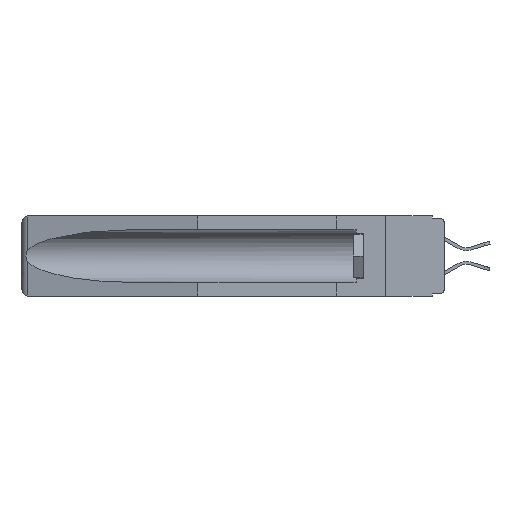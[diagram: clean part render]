
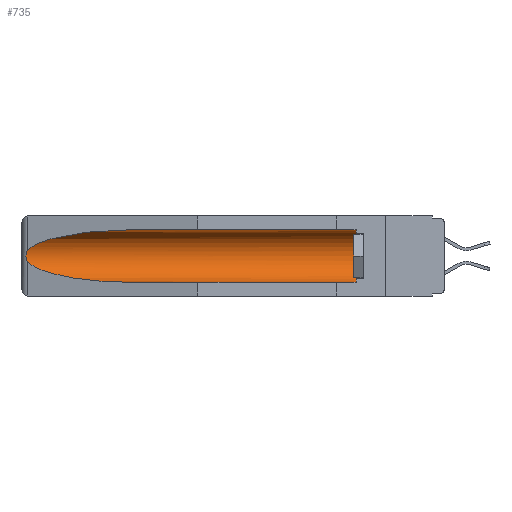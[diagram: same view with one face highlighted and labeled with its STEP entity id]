
A CAD part, left-side view. The second image highlights one B-rep face of the part: STEP entity #735.
In plain terms, the highlighted cylindrical face has radius 2.857 mm (diameter 5.715 mm), a partial arc.
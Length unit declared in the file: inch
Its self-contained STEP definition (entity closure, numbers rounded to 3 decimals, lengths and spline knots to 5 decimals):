
#146 = ORIENTED_EDGE ( 'NONE', *, *, #21408, .T. ) ;
#320 = EDGE_CURVE ( 'NONE', #24030, #10527, #571, .T. ) ;
#353 = CARTESIAN_POINT ( 'NONE',  ( 0.155, 1.07973, -0.284 ) ) ;
#571 = LINE ( 'NONE', #12429, #3613 ) ;
#735 = ADVANCED_FACE ( 'NONE', ( #6229 ), #23232, .F. ) ;
#1528 = CARTESIAN_POINT ( 'NONE',  ( 0.155, 1.07973, -0.284 ) ) ;
#1650 = CARTESIAN_POINT ( 'NONE',  ( 0.26537, 1.52718, -0.19328 ) ) ;
#1743 = CARTESIAN_POINT ( 'NONE',  ( 0.26597, 1.5296, -0.19026 ) ) ;
#1831 = B_SPLINE_CURVE_WITH_KNOTS ( 'NONE', 3,
 ( #9796, #8212, #12398, #12588, #23132, #27302, #14442, #27588, #1743, #1650 ),
 .UNSPECIFIED., .F., .F.,
 ( 4, 2, 2, 2, 4 ),
 ( 0., 0.00029, 0.00058, 0.00087, 0.00117 ),
 .UNSPECIFIED. ) ;
#3613 = VECTOR ( 'NONE', #27330, 39.37008 ) ;
#4956 = AXIS2_PLACEMENT_3D ( 'NONE', #20305, #7686, #22419 ) ;
#5510 = ORIENTED_EDGE ( 'NONE', *, *, #18144, .T. ) ;
#6229 = FACE_OUTER_BOUND ( 'NONE', #10276, .T. ) ;
#6722 = CARTESIAN_POINT ( 'NONE',  ( 0.26537, 1.52718, -0.14972 ) ) ;
#6741 = ORIENTED_EDGE ( 'NONE', *, *, #320, .T. ) ;
#7222 = VERTEX_POINT ( 'NONE', #6722 ) ;
#7345 =( BOUNDED_CURVE ( )  B_SPLINE_CURVE ( 3, ( #22828, #18280, #24866, #1528 ),
 .UNSPECIFIED., .F., .F. ) 
 B_SPLINE_CURVE_WITH_KNOTS ( ( 4, 4 ),
 ( 0.1948, 1.5708 ),
 .UNSPECIFIED. ) 
 CURVE ( )  GEOMETRIC_REPRESENTATION_ITEM ( )  RATIONAL_B_SPLINE_CURVE ( ( 1., 0.848, 0.848, 1. ) ) 
 REPRESENTATION_ITEM ( '' )  );
#7449 = CARTESIAN_POINT ( 'NONE',  ( 0.155, 0.126, -0.284 ) ) ;
#7686 = DIRECTION ( 'NONE',  ( 0., 1., 0. ) ) ;
#8075 = CARTESIAN_POINT ( 'NONE',  ( 0.21114, 1.30732, -0.059 ) ) ;
#8212 = CARTESIAN_POINT ( 'NONE',  ( 0.26597, 1.52961, -0.15275 ) ) ;
#8439 = LINE ( 'NONE', #22333, #11443 ) ;
#9251 = CIRCLE ( 'NONE', #27150, 0.1125 ) ;
#9796 = CARTESIAN_POINT ( 'NONE',  ( 0.26537, 1.52718, -0.14972 ) ) ;
#10276 = EDGE_LOOP ( 'NONE', ( #5510, #10452, #146, #27545, #17547, #6741 ) ) ;
#10452 = ORIENTED_EDGE ( 'NONE', *, *, #19030, .T. ) ;
#10477 = VERTEX_POINT ( 'NONE', #7449 ) ;
#10527 = VERTEX_POINT ( 'NONE', #11981 ) ;
#11443 = VECTOR ( 'NONE', #18132, 39.37008 ) ;
#11981 = CARTESIAN_POINT ( 'NONE',  ( 0.155, 1.07973, -0.059 ) ) ;
#12398 = CARTESIAN_POINT ( 'NONE',  ( 0.26654, 1.53092, -0.15636 ) ) ;
#12429 = CARTESIAN_POINT ( 'NONE',  ( 0.155, -0.30754, -0.059 ) ) ;
#12588 = CARTESIAN_POINT ( 'NONE',  ( 0.2673, 1.5327, -0.16383 ) ) ;
#12639 = CARTESIAN_POINT ( 'NONE',  ( 0.26537, 1.52718, -0.14972 ) ) ;
#12663 = DIRECTION ( 'NONE',  ( 0., -1., 0. ) ) ;
#14442 = CARTESIAN_POINT ( 'NONE',  ( 0.2673, 1.53269, -0.17917 ) ) ;
#14584 = CARTESIAN_POINT ( 'NONE',  ( 0.25451, 1.48313, -0.09465 ) ) ;
#14805 = VERTEX_POINT ( 'NONE', #25664 ) ;
#15906 =( BOUNDED_CURVE ( )  B_SPLINE_CURVE ( 3, ( #20858, #8075, #14584, #12639 ),
 .UNSPECIFIED., .F., .F. ) 
 B_SPLINE_CURVE_WITH_KNOTS ( ( 4, 4 ),
 ( 4.71239, 6.08839 ),
 .UNSPECIFIED. ) 
 CURVE ( )  GEOMETRIC_REPRESENTATION_ITEM ( )  RATIONAL_B_SPLINE_CURVE ( ( 1., 0.848, 0.848, 1. ) ) 
 REPRESENTATION_ITEM ( '' )  );
#16743 = CARTESIAN_POINT ( 'NONE',  ( 0.155, 0.126, -0.059 ) ) ;
#16757 = EDGE_CURVE ( 'NONE', #10477, #25188, #8439, .T. ) ;
#16870 = DIRECTION ( 'NONE',  ( 0., 0., 1. ) ) ;
#17547 = ORIENTED_EDGE ( 'NONE', *, *, #26226, .T. ) ;
#18132 = DIRECTION ( 'NONE',  ( 0., 1., 0. ) ) ;
#18144 = EDGE_CURVE ( 'NONE', #10527, #7222, #15906, .T. ) ;
#18280 = CARTESIAN_POINT ( 'NONE',  ( 0.25451, 1.48313, -0.24835 ) ) ;
#19030 = EDGE_CURVE ( 'NONE', #7222, #14805, #1831, .T. ) ;
#20305 = CARTESIAN_POINT ( 'NONE',  ( 0.155, -0.30754, -0.1715 ) ) ;
#20858 = CARTESIAN_POINT ( 'NONE',  ( 0.155, 1.07973, -0.059 ) ) ;
#21408 = EDGE_CURVE ( 'NONE', #14805, #25188, #7345, .T. ) ;
#22333 = CARTESIAN_POINT ( 'NONE',  ( 0.155, -0.30754, -0.284 ) ) ;
#22419 = DIRECTION ( 'NONE',  ( 0., 0., 1. ) ) ;
#22828 = CARTESIAN_POINT ( 'NONE',  ( 0.26537, 1.52718, -0.19328 ) ) ;
#23132 = CARTESIAN_POINT ( 'NONE',  ( 0.2675, 1.53308, -0.16763 ) ) ;
#23232 = CYLINDRICAL_SURFACE ( 'NONE', #4956, 0.1125 ) ;
#24030 = VERTEX_POINT ( 'NONE', #16743 ) ;
#24866 = CARTESIAN_POINT ( 'NONE',  ( 0.21114, 1.30732, -0.284 ) ) ;
#25188 = VERTEX_POINT ( 'NONE', #353 ) ;
#25328 = CARTESIAN_POINT ( 'NONE',  ( 0.155, 0.126, -0.1715 ) ) ;
#25664 = CARTESIAN_POINT ( 'NONE',  ( 0.26537, 1.52718, -0.19328 ) ) ;
#26226 = EDGE_CURVE ( 'NONE', #10477, #24030, #9251, .T. ) ;
#27150 = AXIS2_PLACEMENT_3D ( 'NONE', #25328, #12663, #16870 ) ;
#27302 = CARTESIAN_POINT ( 'NONE',  ( 0.2675, 1.53308, -0.17534 ) ) ;
#27330 = DIRECTION ( 'NONE',  ( 0., 1., 0. ) ) ;
#27545 = ORIENTED_EDGE ( 'NONE', *, *, #16757, .F. ) ;
#27588 = CARTESIAN_POINT ( 'NONE',  ( 0.26655, 1.53094, -0.18657 ) ) ;
